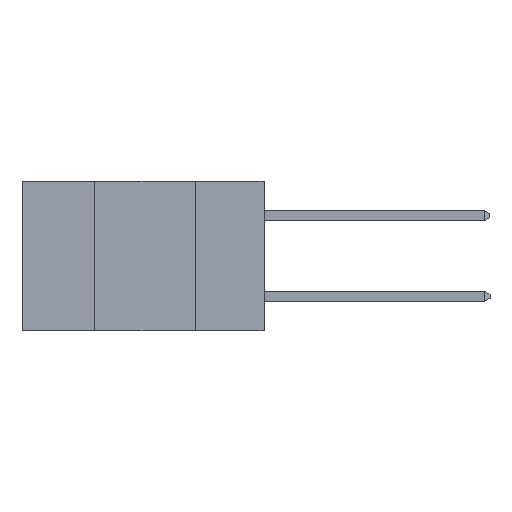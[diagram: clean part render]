
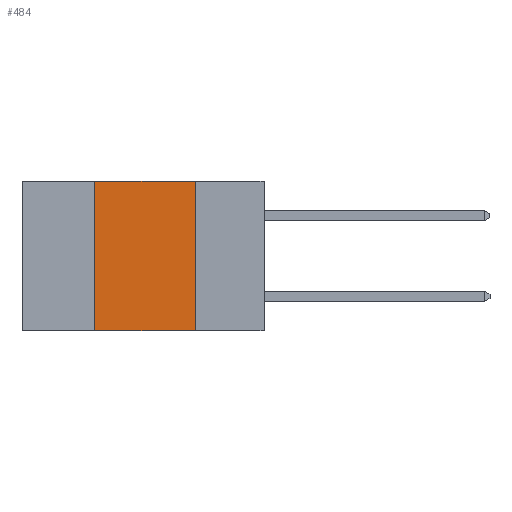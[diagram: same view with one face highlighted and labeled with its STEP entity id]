
A CAD part, left-side view. The second image highlights one B-rep face of the part: STEP entity #484.
In plain terms, the highlighted planar face has unit normal (-1, 0, 0).
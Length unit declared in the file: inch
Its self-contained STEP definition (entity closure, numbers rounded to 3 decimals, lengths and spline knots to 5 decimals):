
#238 = VECTOR ( 'NONE', #7989, 39.37008 ) ;
#256 = ORIENTED_EDGE ( 'NONE', *, *, #1306, .F. ) ;
#330 = EDGE_CURVE ( 'NONE', #7206, #6423, #8184, .T. ) ;
#370 = PLANE ( 'NONE',  #6775 ) ;
#373 = ORIENTED_EDGE ( 'NONE', *, *, #2191, .F. ) ;
#484 = ADVANCED_FACE ( 'NONE', ( #7670 ), #370, .F. ) ;
#699 = LINE ( 'NONE', #4852, #2494 ) ;
#948 = CARTESIAN_POINT ( 'NONE',  ( 0., 0.17, -0.37 ) ) ;
#1090 = VERTEX_POINT ( 'NONE', #948 ) ;
#1306 = EDGE_CURVE ( 'NONE', #6423, #7561, #5005, .T. ) ;
#1386 = VECTOR ( 'NONE', #8503, 39.37008 ) ;
#1629 = CARTESIAN_POINT ( 'NONE',  ( 0., 0.42, -0.37 ) ) ;
#2125 = EDGE_LOOP ( 'NONE', ( #373, #256, #5494, #5553 ) ) ;
#2191 = EDGE_CURVE ( 'NONE', #7561, #1090, #699, .T. ) ;
#2494 = VECTOR ( 'NONE', #4983, 39.37008 ) ;
#2760 = CARTESIAN_POINT ( 'NONE',  ( 0., 0.6, -0.37 ) ) ;
#2768 = VECTOR ( 'NONE', #8024, 39.37008 ) ;
#2825 = CARTESIAN_POINT ( 'NONE',  ( 0., 0.6, 0. ) ) ;
#2994 = LINE ( 'NONE', #2760, #2768 ) ;
#2997 = DIRECTION ( 'NONE',  ( 0., 0., -1. ) ) ;
#3898 = CARTESIAN_POINT ( 'NONE',  ( 0., 0.17, 0. ) ) ;
#4458 = CARTESIAN_POINT ( 'NONE',  ( 0., 0.42, -0.37 ) ) ;
#4852 = CARTESIAN_POINT ( 'NONE',  ( 0., 0.17, -0.37 ) ) ;
#4983 = DIRECTION ( 'NONE',  ( 0., 0., -1. ) ) ;
#5005 = LINE ( 'NONE', #8243, #238 ) ;
#5494 = ORIENTED_EDGE ( 'NONE', *, *, #330, .F. ) ;
#5553 = ORIENTED_EDGE ( 'NONE', *, *, #8518, .T. ) ;
#6423 = VERTEX_POINT ( 'NONE', #7468 ) ;
#6747 = DIRECTION ( 'NONE',  ( 1., 0., 0. ) ) ;
#6775 = AXIS2_PLACEMENT_3D ( 'NONE', #2825, #6747, #2997 ) ;
#7206 = VERTEX_POINT ( 'NONE', #1629 ) ;
#7468 = CARTESIAN_POINT ( 'NONE',  ( 0., 0.42, 0. ) ) ;
#7561 = VERTEX_POINT ( 'NONE', #3898 ) ;
#7670 = FACE_OUTER_BOUND ( 'NONE', #2125, .T. ) ;
#7989 = DIRECTION ( 'NONE',  ( 0., -1., 0. ) ) ;
#8024 = DIRECTION ( 'NONE',  ( 0., -1., 0. ) ) ;
#8184 = LINE ( 'NONE', #4458, #1386 ) ;
#8243 = CARTESIAN_POINT ( 'NONE',  ( 0., 0.6, 0. ) ) ;
#8503 = DIRECTION ( 'NONE',  ( 0., 0., 1. ) ) ;
#8518 = EDGE_CURVE ( 'NONE', #7206, #1090, #2994, .T. ) ;
